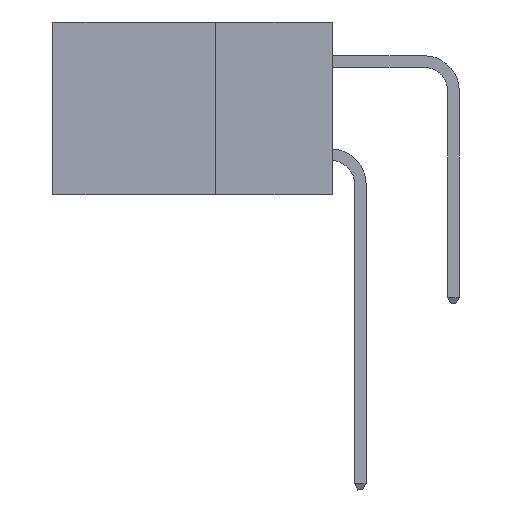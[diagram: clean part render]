
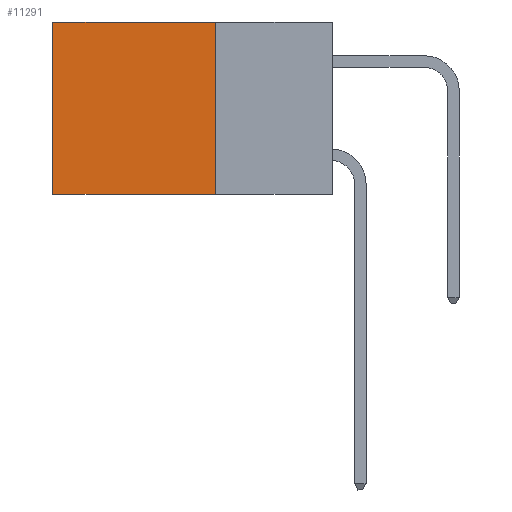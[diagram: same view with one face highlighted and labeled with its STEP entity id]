
A CAD part, left-side view. The second image highlights one B-rep face of the part: STEP entity #11291.
In plain terms, the highlighted planar face has unit normal (-1, 0, 0).
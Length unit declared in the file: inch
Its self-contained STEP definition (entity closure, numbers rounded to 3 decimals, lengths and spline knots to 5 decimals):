
#125 = VECTOR ( 'NONE', #23879, 39.37008 ) ;
#806 = AXIS2_PLACEMENT_3D ( 'NONE', #7803, #21510, #9809 ) ;
#833 = VERTEX_POINT ( 'NONE', #15234 ) ;
#1914 = ORIENTED_EDGE ( 'NONE', *, *, #19412, .F. ) ;
#3654 = VECTOR ( 'NONE', #23100, 39.37008 ) ;
#5502 = CARTESIAN_POINT ( 'NONE',  ( 0.2615, 0.25, -0.37 ) ) ;
#7803 = CARTESIAN_POINT ( 'NONE',  ( 0.2615, 0.25, -0.37 ) ) ;
#7926 = EDGE_CURVE ( 'NONE', #16554, #22811, #9802, .T. ) ;
#8665 = ORIENTED_EDGE ( 'NONE', *, *, #20052, .F. ) ;
#8847 = LINE ( 'NONE', #5502, #3654 ) ;
#9802 = LINE ( 'NONE', #19316, #13757 ) ;
#9809 = DIRECTION ( 'NONE',  ( 0., 0., -1. ) ) ;
#11260 = LINE ( 'NONE', #14235, #125 ) ;
#11291 = ADVANCED_FACE ( 'NONE', ( #25216 ), #11690, .F. ) ;
#11403 = EDGE_LOOP ( 'NONE', ( #21825, #1914, #8665, #17426 ) ) ;
#11536 = DIRECTION ( 'NONE',  ( 0., 1., 0. ) ) ;
#11549 = DIRECTION ( 'NONE',  ( 0., 0., -1. ) ) ;
#11690 = PLANE ( 'NONE',  #806 ) ;
#12830 = VERTEX_POINT ( 'NONE', #21943 ) ;
#13004 = CARTESIAN_POINT ( 'NONE',  ( 0.2615, 0.6, -0.37 ) ) ;
#13757 = VECTOR ( 'NONE', #11549, 39.37008 ) ;
#14235 = CARTESIAN_POINT ( 'NONE',  ( 0.2615, 0.25, 0. ) ) ;
#15234 = CARTESIAN_POINT ( 'NONE',  ( 0.2615, 0.25, 0. ) ) ;
#15966 = EDGE_CURVE ( 'NONE', #833, #16554, #11260, .T. ) ;
#16554 = VERTEX_POINT ( 'NONE', #18334 ) ;
#17426 = ORIENTED_EDGE ( 'NONE', *, *, #15966, .T. ) ;
#18334 = CARTESIAN_POINT ( 'NONE',  ( 0.2615, 0.6, 0. ) ) ;
#18999 = VECTOR ( 'NONE', #11536, 39.37008 ) ;
#19316 = CARTESIAN_POINT ( 'NONE',  ( 0.2615, 0.6, -0.37 ) ) ;
#19412 = EDGE_CURVE ( 'NONE', #12830, #22811, #19616, .T. ) ;
#19616 = LINE ( 'NONE', #23216, #18999 ) ;
#20052 = EDGE_CURVE ( 'NONE', #833, #12830, #8847, .T. ) ;
#21510 = DIRECTION ( 'NONE',  ( 1., 0., 0. ) ) ;
#21825 = ORIENTED_EDGE ( 'NONE', *, *, #7926, .T. ) ;
#21943 = CARTESIAN_POINT ( 'NONE',  ( 0.2615, 0.25, -0.37 ) ) ;
#22811 = VERTEX_POINT ( 'NONE', #13004 ) ;
#23100 = DIRECTION ( 'NONE',  ( 0., 0., -1. ) ) ;
#23216 = CARTESIAN_POINT ( 'NONE',  ( 0.2615, 0.25, -0.37 ) ) ;
#23879 = DIRECTION ( 'NONE',  ( 0., 1., 0. ) ) ;
#25216 = FACE_OUTER_BOUND ( 'NONE', #11403, .T. ) ;
